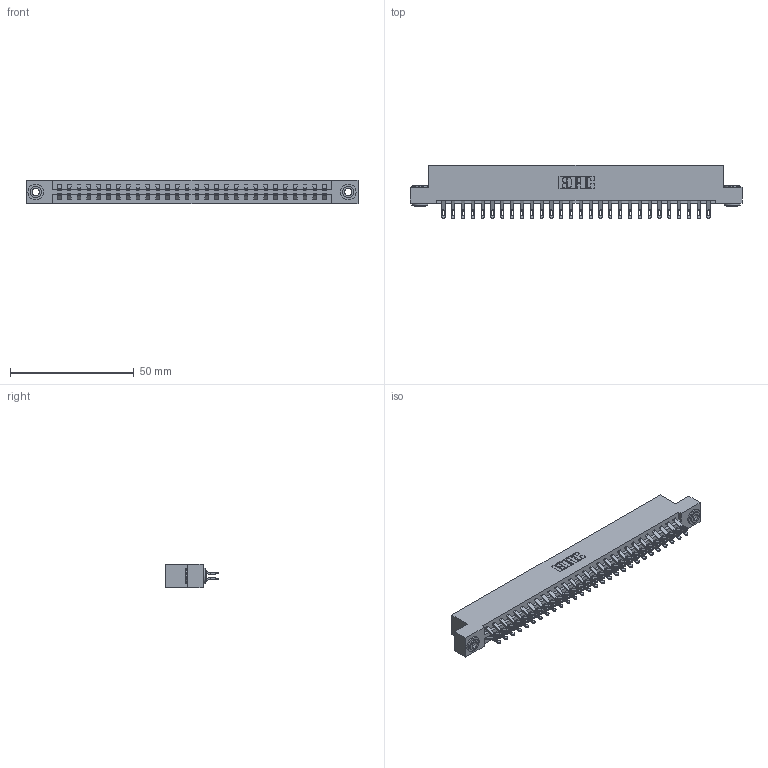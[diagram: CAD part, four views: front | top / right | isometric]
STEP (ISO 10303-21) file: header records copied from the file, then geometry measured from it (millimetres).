
FILE_DESCRIPTION (( 'STEP AP203' ), '1' );
FILE_NAME ('387-056-555-203.STEP', '2018-09-21T00:12:00', ( '' ), ( '' ), 'SwSTEP 2.0', 'SolidWorks 2016', '' );
FILE_SCHEMA (( 'CONFIG_CONTROL_DESIGN' ));
Length unit declared in the file: inch
Products named in the file (4): 337 Part_Flush Mounting Lugs - 0.156 Dia-TH; 345-292-001_555 Tail; 345-250-002_345-250-002-102; 387-056-555-203
Assembly tree (59 placements, depth 2):
  387-056-555-203
    337 Part_Flush Mounting Lugs - 0.156 Dia-TH
    345-292-001_555 Tail  x56
    345-250-002_345-250-002-102  x2
Bounding box: 133.96 x 21.47 x 9.4 mm (x, y, z)
Volume: 14113.2 mm3; surface area: 16655.5 mm2
Topology: 59 solids, 59 shells, 3512 faces, 10971 edges, 7310 vertices
Faces by surface type: plane 2096, cylinder 1408, cone 8
Entity records: 24496 total; most frequent: CARTESIAN_POINT 4147, ORIENTED_EDGE 4046, DIRECTION 3557, EDGE_CURVE 2023, LINE 1851, VECTOR 1851, VERTEX_POINT 1346, AXIS2_PLACEMENT_3D 853
